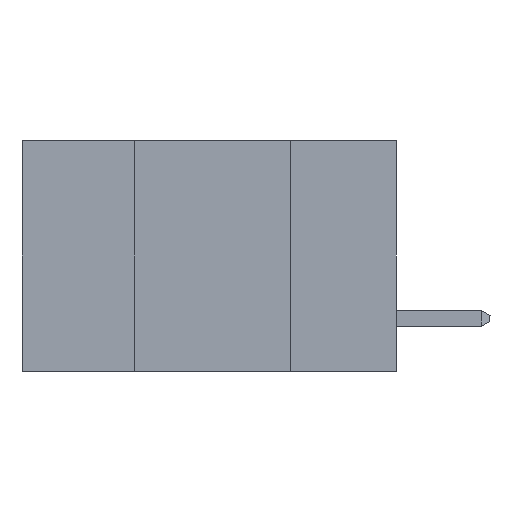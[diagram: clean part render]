
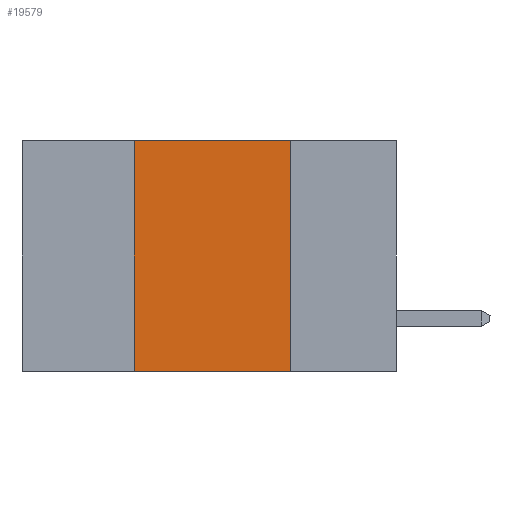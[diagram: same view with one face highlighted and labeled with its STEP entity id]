
A CAD part, left-side view. The second image highlights one B-rep face of the part: STEP entity #19579.
In plain terms, the highlighted planar face has unit normal (-1, 0, 0).
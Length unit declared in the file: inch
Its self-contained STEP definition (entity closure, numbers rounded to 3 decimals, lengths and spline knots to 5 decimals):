
#403 = FACE_OUTER_BOUND ( 'NONE', #24357, .T. ) ;
#658 = DIRECTION ( 'NONE',  ( 0., 0., -1. ) ) ;
#1003 = ORIENTED_EDGE ( 'NONE', *, *, #7902, .F. ) ;
#2944 = DIRECTION ( 'NONE',  ( 0., 0., -1. ) ) ;
#4291 = VECTOR ( 'NONE', #2944, 39.37008 ) ;
#4477 = CARTESIAN_POINT ( 'NONE',  ( 0., 0.42, -0.37 ) ) ;
#5053 = DIRECTION ( 'NONE',  ( 0., 0., 1. ) ) ;
#5396 = VERTEX_POINT ( 'NONE', #5498 ) ;
#5498 = CARTESIAN_POINT ( 'NONE',  ( 0., 0.17, -0.37 ) ) ;
#6274 = PLANE ( 'NONE',  #13818 ) ;
#6540 = ORIENTED_EDGE ( 'NONE', *, *, #16700, .F. ) ;
#7338 = VECTOR ( 'NONE', #21782, 39.37008 ) ;
#7902 = EDGE_CURVE ( 'NONE', #13770, #18405, #16021, .T. ) ;
#8221 = EDGE_CURVE ( 'NONE', #17817, #13770, #18851, .T. ) ;
#9269 = CARTESIAN_POINT ( 'NONE',  ( 0., 0.6, -0.37 ) ) ;
#9921 = ORIENTED_EDGE ( 'NONE', *, *, #8221, .F. ) ;
#9988 = CARTESIAN_POINT ( 'NONE',  ( 0., 0.42, 0. ) ) ;
#11011 = ORIENTED_EDGE ( 'NONE', *, *, #22417, .T. ) ;
#11628 = VECTOR ( 'NONE', #13133, 39.37008 ) ;
#13133 = DIRECTION ( 'NONE',  ( 0., -1., 0. ) ) ;
#13770 = VERTEX_POINT ( 'NONE', #9988 ) ;
#13818 = AXIS2_PLACEMENT_3D ( 'NONE', #21812, #14254, #658 ) ;
#14254 = DIRECTION ( 'NONE',  ( 1., 0., 0. ) ) ;
#16021 = LINE ( 'NONE', #21537, #7338 ) ;
#16684 = LINE ( 'NONE', #20655, #4291 ) ;
#16700 = EDGE_CURVE ( 'NONE', #18405, #5396, #16684, .T. ) ;
#17304 = CARTESIAN_POINT ( 'NONE',  ( 0., 0.42, -0.37 ) ) ;
#17817 = VERTEX_POINT ( 'NONE', #4477 ) ;
#18405 = VERTEX_POINT ( 'NONE', #20878 ) ;
#18851 = LINE ( 'NONE', #17304, #22950 ) ;
#19579 = ADVANCED_FACE ( 'NONE', ( #403 ), #6274, .F. ) ;
#20655 = CARTESIAN_POINT ( 'NONE',  ( 0., 0.17, -0.37 ) ) ;
#20878 = CARTESIAN_POINT ( 'NONE',  ( 0., 0.17, 0. ) ) ;
#21537 = CARTESIAN_POINT ( 'NONE',  ( 0., 0.6, 0. ) ) ;
#21782 = DIRECTION ( 'NONE',  ( 0., -1., 0. ) ) ;
#21812 = CARTESIAN_POINT ( 'NONE',  ( 0., 0.6, 0. ) ) ;
#22417 = EDGE_CURVE ( 'NONE', #17817, #5396, #24955, .T. ) ;
#22950 = VECTOR ( 'NONE', #5053, 39.37008 ) ;
#24357 = EDGE_LOOP ( 'NONE', ( #6540, #1003, #9921, #11011 ) ) ;
#24955 = LINE ( 'NONE', #9269, #11628 ) ;
